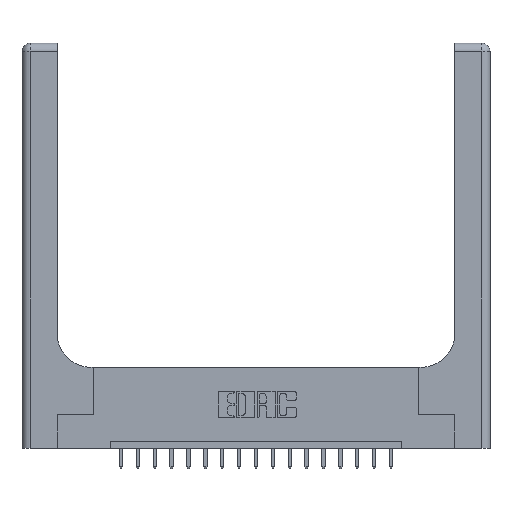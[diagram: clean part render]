
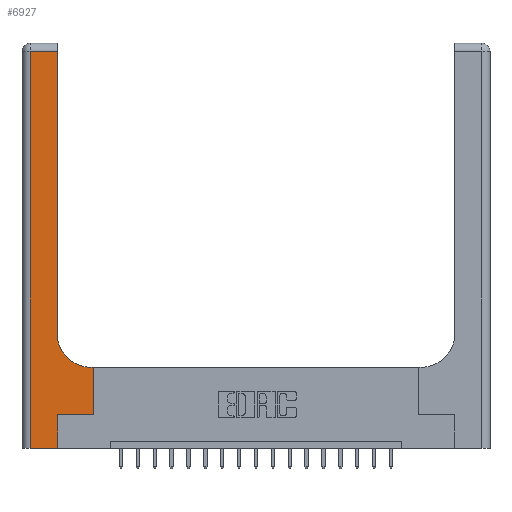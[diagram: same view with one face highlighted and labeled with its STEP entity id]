
A CAD part, top view. The second image highlights one B-rep face of the part: STEP entity #6927.
In plain terms, the highlighted planar face has unit normal (0, 0, 1).
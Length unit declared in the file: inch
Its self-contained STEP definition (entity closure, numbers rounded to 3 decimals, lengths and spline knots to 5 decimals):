
#85 = ORIENTED_EDGE ( 'NONE', *, *, #15882, .T. ) ;
#1148 = CARTESIAN_POINT ( 'NONE',  ( 0.06, 3., 0.37 ) ) ;
#1444 = DIRECTION ( 'NONE',  ( -1., 0., 0. ) ) ;
#1551 = ORIENTED_EDGE ( 'NONE', *, *, #10644, .T. ) ;
#1553 = EDGE_CURVE ( 'NONE', #14001, #11541, #12771, .T. ) ;
#1865 = CARTESIAN_POINT ( 'NONE',  ( 0.528, 0.25, 0.37 ) ) ;
#2080 = VERTEX_POINT ( 'NONE', #11224 ) ;
#2389 = EDGE_LOOP ( 'NONE', ( #14791, #6273, #3590, #8856, #17300, #11292, #1551, #85, #6459 ) ) ;
#2620 = LINE ( 'NONE', #5889, #11189 ) ;
#2723 = EDGE_CURVE ( 'NONE', #11541, #7058, #3159, .T. ) ;
#2817 = DIRECTION ( 'NONE',  ( -1., 0., 0. ) ) ;
#2904 = VECTOR ( 'NONE', #5398, 39.37008 ) ;
#2952 = DIRECTION ( 'NONE',  ( -1., 0., 0. ) ) ;
#3159 = LINE ( 'NONE', #15225, #3162 ) ;
#3162 = VECTOR ( 'NONE', #18603, 39.37008 ) ;
#3294 = CARTESIAN_POINT ( 'NONE',  ( 0.265, 0., 0.37 ) ) ;
#3350 = CARTESIAN_POINT ( 'NONE',  ( 0.26, 2.94, 0.37 ) ) ;
#3443 = EDGE_CURVE ( 'NONE', #15576, #2080, #10322, .T. ) ;
#3590 = ORIENTED_EDGE ( 'NONE', *, *, #3443, .T. ) ;
#3608 = LINE ( 'NONE', #12709, #2904 ) ;
#3955 = LINE ( 'NONE', #5543, #11093 ) ;
#4077 = VERTEX_POINT ( 'NONE', #9889 ) ;
#4272 = EDGE_CURVE ( 'NONE', #2080, #13000, #16526, .T. ) ;
#4330 = LINE ( 'NONE', #10055, #7691 ) ;
#5250 = DIRECTION ( 'NONE',  ( 0., 1., 0. ) ) ;
#5251 = CARTESIAN_POINT ( 'NONE',  ( 0.51, 0.6, 0.37 ) ) ;
#5398 = DIRECTION ( 'NONE',  ( 1., 0., 0. ) ) ;
#5543 = CARTESIAN_POINT ( 'NONE',  ( 0.528, 0.25, 0.37 ) ) ;
#5572 = VECTOR ( 'NONE', #15229, 39.37008 ) ;
#5889 = CARTESIAN_POINT ( 'NONE',  ( 0., 2.94, 0.37 ) ) ;
#5957 = AXIS2_PLACEMENT_3D ( 'NONE', #7389, #17911, #2952 ) ;
#6273 = ORIENTED_EDGE ( 'NONE', *, *, #16276, .T. ) ;
#6459 = ORIENTED_EDGE ( 'NONE', *, *, #1553, .T. ) ;
#6927 = ADVANCED_FACE ( 'NONE', ( #8881 ), #19487, .F. ) ;
#7058 = VERTEX_POINT ( 'NONE', #3350 ) ;
#7112 = VERTEX_POINT ( 'NONE', #1865 ) ;
#7389 = CARTESIAN_POINT ( 'NONE',  ( 0., 3., 0.37 ) ) ;
#7691 = VECTOR ( 'NONE', #1444, 39.37008 ) ;
#7905 = CARTESIAN_POINT ( 'NONE',  ( 0.265, 0., 0.37 ) ) ;
#8260 = CARTESIAN_POINT ( 'NONE',  ( 0.51, 0.85, 0.37 ) ) ;
#8856 = ORIENTED_EDGE ( 'NONE', *, *, #4272, .T. ) ;
#8881 = FACE_OUTER_BOUND ( 'NONE', #2389, .T. ) ;
#9889 = CARTESIAN_POINT ( 'NONE',  ( 0.265, 0.25, 0.37 ) ) ;
#10055 = CARTESIAN_POINT ( 'NONE',  ( 0.26, 0.6, 0.37 ) ) ;
#10322 = LINE ( 'NONE', #1148, #16275 ) ;
#10644 = EDGE_CURVE ( 'NONE', #7112, #14285, #3955, .T. ) ;
#10759 = CARTESIAN_POINT ( 'NONE',  ( 0., 0., 0.37 ) ) ;
#11066 = LINE ( 'NONE', #7905, #13988 ) ;
#11093 = VECTOR ( 'NONE', #16035, 39.37008 ) ;
#11189 = VECTOR ( 'NONE', #2817, 39.37008 ) ;
#11224 = CARTESIAN_POINT ( 'NONE',  ( 0.06, 0., 0.37 ) ) ;
#11292 = ORIENTED_EDGE ( 'NONE', *, *, #11472, .T. ) ;
#11472 = EDGE_CURVE ( 'NONE', #4077, #7112, #3608, .T. ) ;
#11541 = VERTEX_POINT ( 'NONE', #15980 ) ;
#11814 = DIRECTION ( 'NONE',  ( 0., -1., 0. ) ) ;
#12384 = EDGE_CURVE ( 'NONE', #13000, #4077, #11066, .T. ) ;
#12451 = AXIS2_PLACEMENT_3D ( 'NONE', #8260, #14108, #18672 ) ;
#12709 = CARTESIAN_POINT ( 'NONE',  ( 0.265, 0.25, 0.37 ) ) ;
#12771 = CIRCLE ( 'NONE', #12451, 0.25 ) ;
#13000 = VERTEX_POINT ( 'NONE', #3294 ) ;
#13988 = VECTOR ( 'NONE', #5250, 39.37008 ) ;
#14001 = VERTEX_POINT ( 'NONE', #5251 ) ;
#14108 = DIRECTION ( 'NONE',  ( 0., 0., -1. ) ) ;
#14285 = VERTEX_POINT ( 'NONE', #18289 ) ;
#14791 = ORIENTED_EDGE ( 'NONE', *, *, #2723, .T. ) ;
#15225 = CARTESIAN_POINT ( 'NONE',  ( 0.26, 3., 0.37 ) ) ;
#15229 = DIRECTION ( 'NONE',  ( 1., 0., 0. ) ) ;
#15576 = VERTEX_POINT ( 'NONE', #16710 ) ;
#15882 = EDGE_CURVE ( 'NONE', #14285, #14001, #4330, .T. ) ;
#15980 = CARTESIAN_POINT ( 'NONE',  ( 0.26, 0.85, 0.37 ) ) ;
#16035 = DIRECTION ( 'NONE',  ( 0., 1., 0. ) ) ;
#16275 = VECTOR ( 'NONE', #11814, 39.37008 ) ;
#16276 = EDGE_CURVE ( 'NONE', #7058, #15576, #2620, .T. ) ;
#16526 = LINE ( 'NONE', #10759, #5572 ) ;
#16710 = CARTESIAN_POINT ( 'NONE',  ( 0.06, 2.94, 0.37 ) ) ;
#17300 = ORIENTED_EDGE ( 'NONE', *, *, #12384, .T. ) ;
#17911 = DIRECTION ( 'NONE',  ( 0., 0., -1. ) ) ;
#18289 = CARTESIAN_POINT ( 'NONE',  ( 0.528, 0.6, 0.37 ) ) ;
#18603 = DIRECTION ( 'NONE',  ( 0., 1., 0. ) ) ;
#18672 = DIRECTION ( 'NONE',  ( 1., 0., 0. ) ) ;
#19487 = PLANE ( 'NONE',  #5957 ) ;
